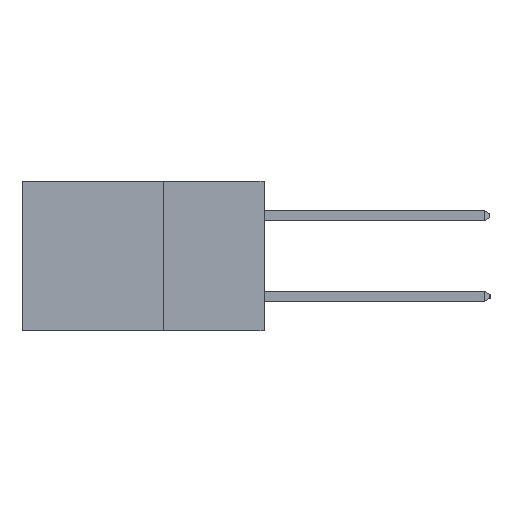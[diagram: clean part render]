
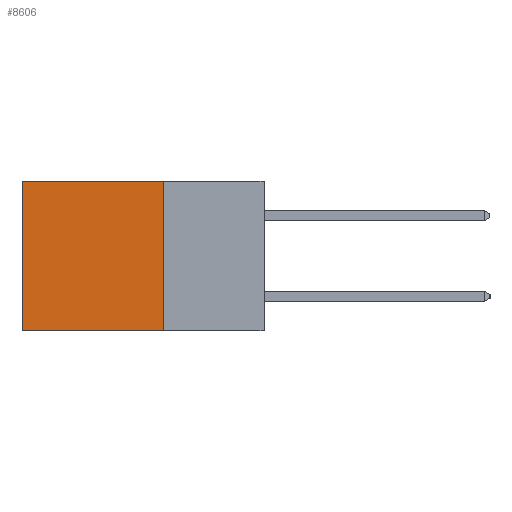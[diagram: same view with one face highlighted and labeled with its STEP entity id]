
A CAD part, left-side view. The second image highlights one B-rep face of the part: STEP entity #8606.
In plain terms, the highlighted planar face has unit normal (-1, 0, 0).
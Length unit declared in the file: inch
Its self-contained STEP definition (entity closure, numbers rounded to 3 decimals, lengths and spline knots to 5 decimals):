
#256 = EDGE_CURVE ( 'NONE', #11939, #5725, #4305, .T. ) ;
#992 = DIRECTION ( 'NONE',  ( 0., 0., -1. ) ) ;
#1043 = CARTESIAN_POINT ( 'NONE',  ( 0.2615, 0.25, -0.37 ) ) ;
#1048 = PLANE ( 'NONE',  #6005 ) ;
#1298 = DIRECTION ( 'NONE',  ( 1., 0., 0. ) ) ;
#1404 = EDGE_LOOP ( 'NONE', ( #2352, #6580, #3262, #7718 ) ) ;
#1408 = VECTOR ( 'NONE', #8866, 39.37008 ) ;
#1581 = VERTEX_POINT ( 'NONE', #10801 ) ;
#2352 = ORIENTED_EDGE ( 'NONE', *, *, #8168, .T. ) ;
#2363 = VERTEX_POINT ( 'NONE', #10099 ) ;
#2768 = CARTESIAN_POINT ( 'NONE',  ( 0.2615, 0.6, -0.37 ) ) ;
#2775 = CARTESIAN_POINT ( 'NONE',  ( 0.2615, 0.25, -0.37 ) ) ;
#2799 = DIRECTION ( 'NONE',  ( 0., 0., -1. ) ) ;
#2808 = EDGE_CURVE ( 'NONE', #2363, #11939, #8737, .T. ) ;
#3206 = FACE_OUTER_BOUND ( 'NONE', #1404, .T. ) ;
#3262 = ORIENTED_EDGE ( 'NONE', *, *, #2808, .F. ) ;
#3409 = VECTOR ( 'NONE', #2799, 39.37008 ) ;
#3509 = EDGE_CURVE ( 'NONE', #2363, #1581, #5448, .T. ) ;
#4305 = LINE ( 'NONE', #8728, #1408 ) ;
#5213 = CARTESIAN_POINT ( 'NONE',  ( 0.2615, 0.25, 0. ) ) ;
#5384 = DIRECTION ( 'NONE',  ( 0., 1., 0. ) ) ;
#5448 = LINE ( 'NONE', #5213, #7840 ) ;
#5725 = VERTEX_POINT ( 'NONE', #11381 ) ;
#6005 = AXIS2_PLACEMENT_3D ( 'NONE', #1043, #1298, #992 ) ;
#6580 = ORIENTED_EDGE ( 'NONE', *, *, #256, .F. ) ;
#6932 = DIRECTION ( 'NONE',  ( 0., 0., -1. ) ) ;
#7718 = ORIENTED_EDGE ( 'NONE', *, *, #3509, .T. ) ;
#7840 = VECTOR ( 'NONE', #5384, 39.37008 ) ;
#8168 = EDGE_CURVE ( 'NONE', #1581, #5725, #8619, .T. ) ;
#8606 = ADVANCED_FACE ( 'NONE', ( #3206 ), #1048, .F. ) ;
#8619 = LINE ( 'NONE', #2768, #3409 ) ;
#8728 = CARTESIAN_POINT ( 'NONE',  ( 0.2615, 0.25, -0.37 ) ) ;
#8737 = LINE ( 'NONE', #2775, #10868 ) ;
#8866 = DIRECTION ( 'NONE',  ( 0., 1., 0. ) ) ;
#10099 = CARTESIAN_POINT ( 'NONE',  ( 0.2615, 0.25, 0. ) ) ;
#10801 = CARTESIAN_POINT ( 'NONE',  ( 0.2615, 0.6, 0. ) ) ;
#10868 = VECTOR ( 'NONE', #6932, 39.37008 ) ;
#11381 = CARTESIAN_POINT ( 'NONE',  ( 0.2615, 0.6, -0.37 ) ) ;
#11939 = VERTEX_POINT ( 'NONE', #11987 ) ;
#11987 = CARTESIAN_POINT ( 'NONE',  ( 0.2615, 0.25, -0.37 ) ) ;
